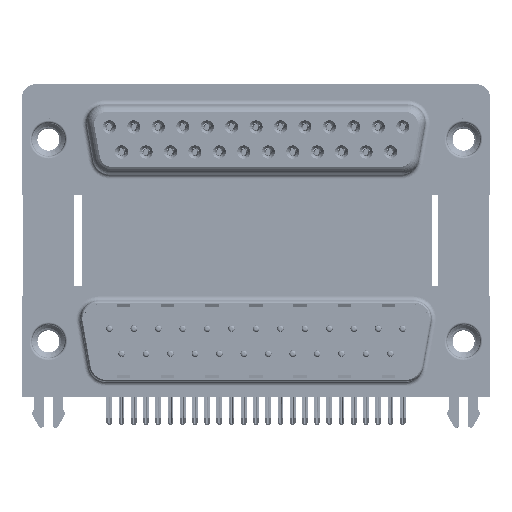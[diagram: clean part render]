
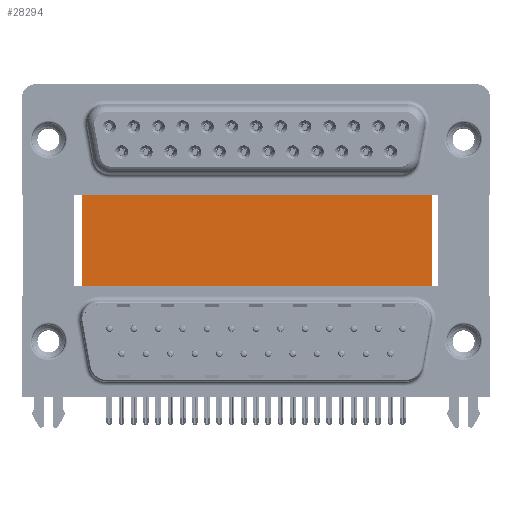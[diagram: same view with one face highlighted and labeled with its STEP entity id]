
A CAD part, top view. The second image highlights one B-rep face of the part: STEP entity #28294.
In plain terms, the highlighted planar face has unit normal (0, 0, 1).
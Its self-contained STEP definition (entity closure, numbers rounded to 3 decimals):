
#424 = PLANE ( 'NONE',  #42625 ) ;
#1686 = VERTEX_POINT ( 'NONE', #13297 ) ;
#1781 = EDGE_LOOP ( 'NONE', ( #4285, #42561, #10955, #6314 ) ) ;
#4285 = ORIENTED_EDGE ( 'NONE', *, *, #54389, .T. ) ;
#5317 = EDGE_CURVE ( 'NONE', #39502, #11605, #27574, .T. ) ;
#6314 = ORIENTED_EDGE ( 'NONE', *, *, #43846, .T. ) ;
#9439 = DIRECTION ( 'NONE',  ( 0., 0., -1. ) ) ;
#10955 = ORIENTED_EDGE ( 'NONE', *, *, #27568, .F. ) ;
#11559 = VERTEX_POINT ( 'NONE', #55471 ) ;
#11605 = VERTEX_POINT ( 'NONE', #38878 ) ;
#13297 = CARTESIAN_POINT ( 'NONE',  ( 3.79, -3.735, -12. ) ) ;
#15214 = VECTOR ( 'NONE', #50256, 1000. ) ;
#22463 = DIRECTION ( 'NONE',  ( 1., 0., 0. ) ) ;
#24050 = CARTESIAN_POINT ( 'NONE',  ( 43.43, 16.585, -12. ) ) ;
#25888 = LINE ( 'NONE', #39590, #47386 ) ;
#27022 = CARTESIAN_POINT ( 'NONE',  ( 43.43, 16.585, -12. ) ) ;
#27568 = EDGE_CURVE ( 'NONE', #11559, #39502, #35879, .T. ) ;
#27574 = LINE ( 'NONE', #24050, #15214 ) ;
#28139 = VECTOR ( 'NONE', #32678, 1000. ) ;
#28294 = ADVANCED_FACE ( 'NONE', ( #40326 ), #424, .F. ) ;
#31562 = CARTESIAN_POINT ( 'NONE',  ( 3.79, 16.585, -12. ) ) ;
#32678 = DIRECTION ( 'NONE',  ( 1., 0., 0. ) ) ;
#35879 = LINE ( 'NONE', #36153, #40762 ) ;
#36153 = CARTESIAN_POINT ( 'NONE',  ( 3.79, 16.585, -12. ) ) ;
#36503 = CARTESIAN_POINT ( 'NONE',  ( 3.79, -3.735, -12. ) ) ;
#38878 = CARTESIAN_POINT ( 'NONE',  ( 43.43, -3.735, -12. ) ) ;
#39502 = VERTEX_POINT ( 'NONE', #27022 ) ;
#39590 = CARTESIAN_POINT ( 'NONE',  ( 3.79, 16.585, -12. ) ) ;
#40326 = FACE_OUTER_BOUND ( 'NONE', #1781, .T. ) ;
#40762 = VECTOR ( 'NONE', #22463, 1000. ) ;
#42561 = ORIENTED_EDGE ( 'NONE', *, *, #5317, .F. ) ;
#42625 = AXIS2_PLACEMENT_3D ( 'NONE', #31562, #9439, #44987 ) ;
#43846 = EDGE_CURVE ( 'NONE', #11559, #1686, #25888, .T. ) ;
#44987 = DIRECTION ( 'NONE',  ( -1., 0., 0. ) ) ;
#46084 = LINE ( 'NONE', #36503, #28139 ) ;
#47386 = VECTOR ( 'NONE', #49164, 1000. ) ;
#49164 = DIRECTION ( 'NONE',  ( 0., -1., 0. ) ) ;
#50256 = DIRECTION ( 'NONE',  ( 0., -1., 0. ) ) ;
#54389 = EDGE_CURVE ( 'NONE', #1686, #11605, #46084, .T. ) ;
#55471 = CARTESIAN_POINT ( 'NONE',  ( 3.79, 16.585, -12. ) ) ;
